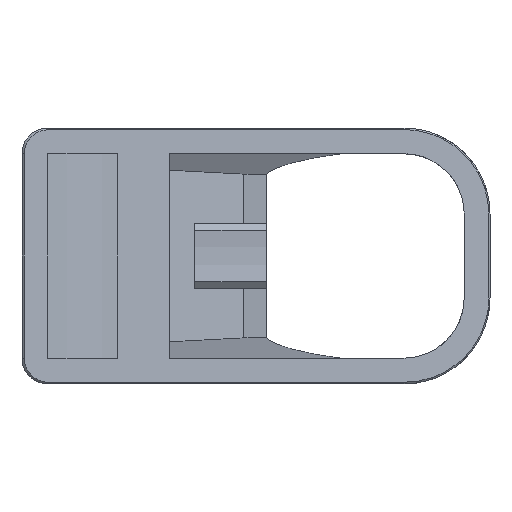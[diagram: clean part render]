
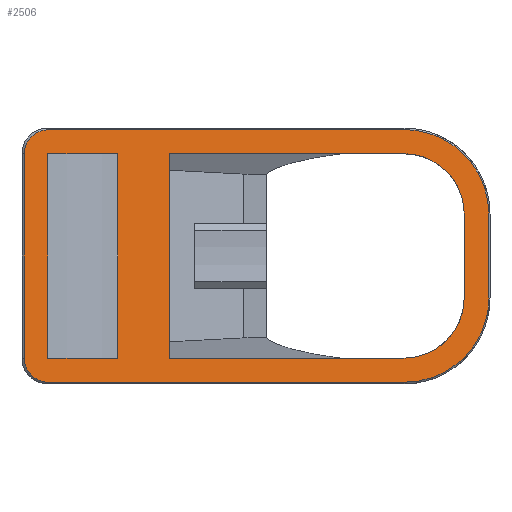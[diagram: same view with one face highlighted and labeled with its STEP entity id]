
A CAD part, front view. The second image highlights one B-rep face of the part: STEP entity #2506.
In plain terms, the highlighted planar face has unit normal (0.309, -0.951, 0).
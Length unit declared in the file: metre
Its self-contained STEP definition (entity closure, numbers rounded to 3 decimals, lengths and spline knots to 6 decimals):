
#103=ELLIPSE('',#2674,0.00736,0.007);
#104=ELLIPSE('',#2675,0.00736,0.007);
#184=B_SPLINE_CURVE_WITH_KNOTS('',3,(#3605,#3606,#3607,#3608,#3609,#3610,
#3611,#3612,#3613),.UNSPECIFIED.,.F.,.F.,(4,1,1,1,1,1,4),(0.,0.125,0.25,
0.5,0.75,0.875,1.),.UNSPECIFIED.);
#185=B_SPLINE_CURVE_WITH_KNOTS('',3,(#3618,#3619,#3620,#3621,#3622),
 .UNSPECIFIED.,.F.,.F.,(4,1,4),(0.,0.5,1.),.UNSPECIFIED.);
#186=B_SPLINE_CURVE_WITH_KNOTS('',3,(#3626,#3627,#3628,#3629,#3630),
 .UNSPECIFIED.,.F.,.F.,(4,1,4),(0.,0.5,1.),.UNSPECIFIED.);
#187=B_SPLINE_CURVE_WITH_KNOTS('',3,(#3634,#3635,#3636,#3637,#3638,#3639,
#3640,#3641),.UNSPECIFIED.,.F.,.F.,(4,1,1,1,1,4),(0.,0.125,0.25,0.5,0.75,
1.),.UNSPECIFIED.);
#371=ORIENTED_EDGE('',*,*,#1143,.T.);
#372=ORIENTED_EDGE('',*,*,#1144,.T.);
#373=ORIENTED_EDGE('',*,*,#1145,.T.);
#374=ORIENTED_EDGE('',*,*,#1146,.T.);
#375=ORIENTED_EDGE('',*,*,#1147,.T.);
#376=ORIENTED_EDGE('',*,*,#1148,.T.);
#377=ORIENTED_EDGE('',*,*,#1149,.T.);
#378=ORIENTED_EDGE('',*,*,#1150,.T.);
#379=ORIENTED_EDGE('',*,*,#1151,.F.);
#380=ORIENTED_EDGE('',*,*,#1152,.T.);
#381=ORIENTED_EDGE('',*,*,#1127,.F.);
#382=ORIENTED_EDGE('',*,*,#1153,.F.);
#383=ORIENTED_EDGE('',*,*,#1154,.F.);
#384=ORIENTED_EDGE('',*,*,#1155,.T.);
#385=ORIENTED_EDGE('',*,*,#1156,.F.);
#386=ORIENTED_EDGE('',*,*,#1157,.F.);
#387=ORIENTED_EDGE('',*,*,#1158,.T.);
#388=ORIENTED_EDGE('',*,*,#1159,.T.);
#1127=EDGE_CURVE('',#1513,#1514,#1716,.T.);
#1143=EDGE_CURVE('',#1529,#1530,#184,.T.);
#1144=EDGE_CURVE('',#1530,#1531,#1731,.T.);
#1145=EDGE_CURVE('',#1531,#1532,#185,.T.);
#1146=EDGE_CURVE('',#1532,#1533,#1732,.T.);
#1147=EDGE_CURVE('',#1533,#1534,#186,.T.);
#1148=EDGE_CURVE('',#1534,#1535,#1733,.T.);
#1149=EDGE_CURVE('',#1535,#1536,#187,.T.);
#1150=EDGE_CURVE('',#1536,#1529,#1734,.T.);
#1151=EDGE_CURVE('',#1537,#1538,#103,.T.);
#1152=EDGE_CURVE('',#1537,#1514,#1735,.T.);
#1153=EDGE_CURVE('',#1539,#1513,#1736,.T.);
#1154=EDGE_CURVE('',#1540,#1539,#104,.T.);
#1155=EDGE_CURVE('',#1540,#1538,#1737,.T.);
#1156=EDGE_CURVE('',#1541,#1542,#1738,.T.);
#1157=EDGE_CURVE('',#1543,#1541,#1739,.T.);
#1158=EDGE_CURVE('',#1543,#1544,#1740,.T.);
#1159=EDGE_CURVE('',#1544,#1542,#1741,.T.);
#1513=VERTEX_POINT('',#3566);
#1514=VERTEX_POINT('',#3568);
#1529=VERTEX_POINT('',#3614);
#1530=VERTEX_POINT('',#3615);
#1531=VERTEX_POINT('',#3617);
#1532=VERTEX_POINT('',#3623);
#1533=VERTEX_POINT('',#3625);
#1534=VERTEX_POINT('',#3631);
#1535=VERTEX_POINT('',#3633);
#1536=VERTEX_POINT('',#3642);
#1537=VERTEX_POINT('',#3645);
#1538=VERTEX_POINT('',#3646);
#1539=VERTEX_POINT('',#3649);
#1540=VERTEX_POINT('',#3651);
#1541=VERTEX_POINT('',#3654);
#1542=VERTEX_POINT('',#3655);
#1543=VERTEX_POINT('',#3657);
#1544=VERTEX_POINT('',#3659);
#1716=LINE('',#3567,#1936);
#1731=LINE('',#3616,#1951);
#1732=LINE('',#3624,#1952);
#1733=LINE('',#3632,#1953);
#1734=LINE('',#3643,#1954);
#1735=LINE('',#3647,#1955);
#1736=LINE('',#3648,#1956);
#1737=LINE('',#3652,#1957);
#1738=LINE('',#3653,#1958);
#1739=LINE('',#3656,#1959);
#1740=LINE('',#3658,#1960);
#1741=LINE('',#3660,#1961);
#1936=VECTOR('',#2864,1.);
#1951=VECTOR('',#2887,1.);
#1952=VECTOR('',#2888,1.);
#1953=VECTOR('',#2889,1.);
#1954=VECTOR('',#2890,1.);
#1955=VECTOR('',#2893,1.);
#1956=VECTOR('',#2894,1.);
#1957=VECTOR('',#2897,1.);
#1958=VECTOR('',#2898,1.);
#1959=VECTOR('',#2899,1.);
#1960=VECTOR('',#2900,1.);
#1961=VECTOR('',#2901,1.);
#2123=EDGE_LOOP('',(#371,#372,#373,#374,#375,#376,#377,#378));
#2124=EDGE_LOOP('',(#379,#380,#381,#382,#383,#384));
#2125=EDGE_LOOP('',(#385,#386,#387,#388));
#2283=FACE_BOUND('',#2123,.T.);
#2284=FACE_BOUND('',#2124,.T.);
#2285=FACE_BOUND('',#2125,.T.);
#2438=PLANE('',#2673);
#2506=ADVANCED_FACE('',(#2283,#2284,#2285),#2438,.T.);
#2673=AXIS2_PLACEMENT_3D('',#3604,#2885,#2886);
#2674=AXIS2_PLACEMENT_3D('',#3644,#2891,#2892);
#2675=AXIS2_PLACEMENT_3D('',#3650,#2895,#2896);
#2864=DIRECTION('',(0.,0.,-1.));
#2885=DIRECTION('',(0.309,-0.951,0.));
#2886=DIRECTION('',(0.951,0.309,0.));
#2887=DIRECTION('',(-0.951,-0.309,0.));
#2888=DIRECTION('',(0.,0.,-1.));
#2889=DIRECTION('',(0.951,0.309,0.));
#2890=DIRECTION('',(0.,0.,1.));
#2891=DIRECTION('',(0.309,-0.951,0.));
#2892=DIRECTION('',(0.951,0.309,0.));
#2893=DIRECTION('',(-0.951,-0.309,0.));
#2894=DIRECTION('',(-0.951,-0.309,0.));
#2895=DIRECTION('',(0.309,-0.951,0.));
#2896=DIRECTION('',(-0.951,-0.309,0.));
#2897=DIRECTION('',(0.,0.,-1.));
#2898=DIRECTION('',(0.,0.,-1.));
#2899=DIRECTION('',(-0.951,-0.309,0.));
#2900=DIRECTION('',(0.,0.,-1.));
#2901=DIRECTION('',(-0.951,-0.309,0.));
#3566=CARTESIAN_POINT('',(-0.01099,-0.034024,0.02675));
#3567=CARTESIAN_POINT('',(-0.01099,-0.034024,0.02975));
#3568=CARTESIAN_POINT('',(-0.01099,-0.034024,0.003));
#3604=CARTESIAN_POINT('',(0.00616,-0.028451,0.02975));
#3605=CARTESIAN_POINT('',(0.026172,-0.021949,0.01975));
#3606=CARTESIAN_POINT('',(0.026172,-0.021949,0.020399));
#3607=CARTESIAN_POINT('',(0.026049,-0.021989,0.021669));
#3608=CARTESIAN_POINT('',(0.025295,-0.022234,0.024144));
#3609=CARTESIAN_POINT('',(0.023482,-0.022823,0.02686));
#3610=CARTESIAN_POINT('',(0.020766,-0.023706,0.028674));
#3611=CARTESIAN_POINT('',(0.018291,-0.02451,0.029428));
#3612=CARTESIAN_POINT('',(0.017021,-0.024923,0.02955));
#3613=CARTESIAN_POINT('',(0.016372,-0.025133,0.02955));
#3614=CARTESIAN_POINT('',(0.026172,-0.021949,0.01975));
#3615=CARTESIAN_POINT('',(0.016372,-0.025133,0.02955));
#3616=CARTESIAN_POINT('',(0.00616,-0.028451,0.02955));
#3617=CARTESIAN_POINT('',(-0.025034,-0.038587,0.02955));
#3618=CARTESIAN_POINT('',(-0.025034,-0.038587,0.02955));
#3619=CARTESIAN_POINT('',(-0.025766,-0.038825,0.029553));
#3620=CARTESIAN_POINT('',(-0.027227,-0.039299,0.028942));
#3621=CARTESIAN_POINT('',(-0.027837,-0.039498,0.027483));
#3622=CARTESIAN_POINT('',(-0.027834,-0.039497,0.02675));
#3623=CARTESIAN_POINT('',(-0.027834,-0.039497,0.02675));
#3624=CARTESIAN_POINT('',(-0.027834,-0.039497,0.02975));
#3625=CARTESIAN_POINT('',(-0.027834,-0.039497,0.003));
#3626=CARTESIAN_POINT('',(-0.027834,-0.039497,0.003));
#3627=CARTESIAN_POINT('',(-0.027837,-0.039498,0.002268));
#3628=CARTESIAN_POINT('',(-0.027226,-0.039299,0.000808));
#3629=CARTESIAN_POINT('',(-0.025767,-0.038825,0.000197));
#3630=CARTESIAN_POINT('',(-0.025034,-0.038587,0.0002));
#3631=CARTESIAN_POINT('',(-0.025034,-0.038587,0.0002));
#3632=CARTESIAN_POINT('',(0.01631,-0.025153,0.0002));
#3633=CARTESIAN_POINT('',(0.016372,-0.025133,0.0002));
#3634=CARTESIAN_POINT('',(0.016372,-0.025133,0.0002));
#3635=CARTESIAN_POINT('',(0.017021,-0.024923,0.0002));
#3636=CARTESIAN_POINT('',(0.018291,-0.02451,0.000322));
#3637=CARTESIAN_POINT('',(0.020766,-0.023706,0.001077));
#3638=CARTESIAN_POINT('',(0.023481,-0.022824,0.002887));
#3639=CARTESIAN_POINT('',(0.025661,-0.022115,0.00616));
#3640=CARTESIAN_POINT('',(0.026172,-0.021949,0.008702));
#3641=CARTESIAN_POINT('',(0.026172,-0.021949,0.01));
#3642=CARTESIAN_POINT('',(0.026172,-0.021949,0.01));
#3643=CARTESIAN_POINT('',(0.026172,-0.021949,0.01975));
#3644=CARTESIAN_POINT('',(0.01631,-0.025153,0.01));
#3645=CARTESIAN_POINT('',(0.01631,-0.025153,0.003));
#3646=CARTESIAN_POINT('',(0.02331,-0.022879,0.01));
#3647=CARTESIAN_POINT('',(0.00616,-0.028451,0.003));
#3648=CARTESIAN_POINT('',(0.00616,-0.028451,0.02675));
#3649=CARTESIAN_POINT('',(0.01631,-0.025153,0.02675));
#3650=CARTESIAN_POINT('',(0.01631,-0.025153,0.01975));
#3651=CARTESIAN_POINT('',(0.02331,-0.022879,0.01975));
#3652=CARTESIAN_POINT('',(0.02331,-0.022879,0.02975));
#3653=CARTESIAN_POINT('',(-0.025096,-0.038607,0.02975));
#3654=CARTESIAN_POINT('',(-0.025096,-0.038607,0.02675));
#3655=CARTESIAN_POINT('',(-0.025096,-0.038607,0.003));
#3656=CARTESIAN_POINT('',(-0.021043,-0.03729,0.02675));
#3657=CARTESIAN_POINT('',(-0.01699,-0.035973,0.02675));
#3658=CARTESIAN_POINT('',(-0.01699,-0.035973,0.02975));
#3659=CARTESIAN_POINT('',(-0.01699,-0.035973,0.003));
#3660=CARTESIAN_POINT('',(-0.021043,-0.03729,0.003));
